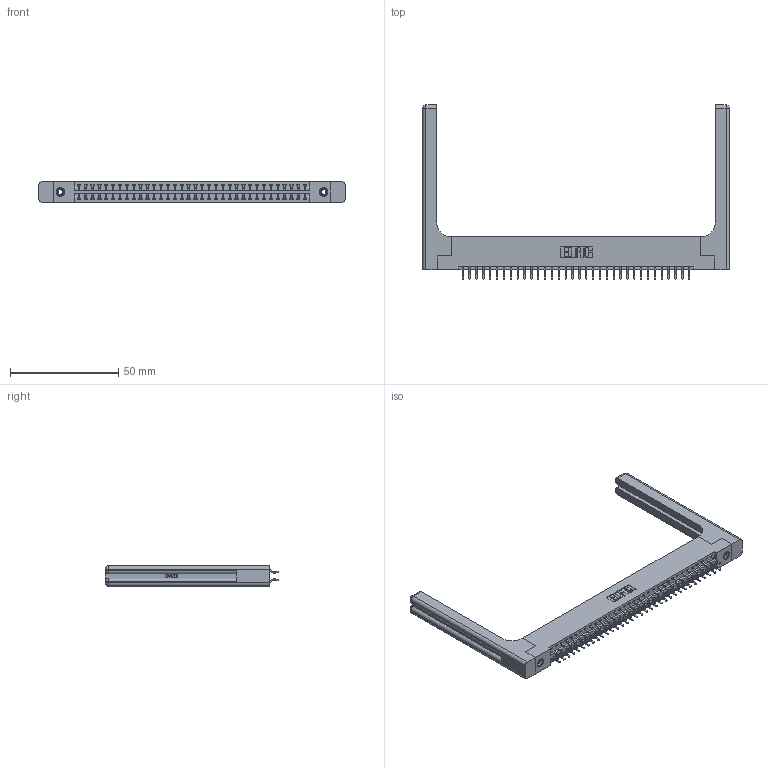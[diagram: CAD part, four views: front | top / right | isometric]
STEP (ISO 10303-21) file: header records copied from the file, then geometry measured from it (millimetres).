
FILE_DESCRIPTION (( 'STEP AP203' ), '1' );
FILE_NAME ('346-068-556-258.STEP', '2022-05-24T19:52:04', ( '' ), ( '' ), 'SwSTEP 2.0', 'SolidWorks 2020', '' );
FILE_SCHEMA (( 'CONFIG_CONTROL_DESIGN' ));
Length unit declared in the file: inch
Products named in the file (5): 346 Part_Flush Mounting Lugs - 0.156 Dia-TH; 346-068-556-258; 346-220-058_345-220-058; 345-292-001_556 Tail; 345-250-001_345-250-001-102
Assembly tree (73 placements, depth 2):
  346-068-556-258
    346 Part_Flush Mounting Lugs - 0.156 Dia-TH
    345-292-001_556 Tail  x68
    345-250-001_345-250-001-102  x2
    346-220-058_345-220-058  x2
Bounding box: 142.01 x 80.53 x 9.4 mm (x, y, z)
Volume: 21259.2 mm3; surface area: 23739.3 mm2
Topology: 73 solids, 73 shells, 4336 faces, 12795 edges, 8418 vertices
Faces by surface type: plane 2890, cylinder 1386, bspline 36, cone 12, sphere 8, torus 4
Entity records: 29084 total; most frequent: CARTESIAN_POINT 5831, ORIENTED_EDGE 4548, DIRECTION 4110, EDGE_CURVE 2274, VECTOR 1906, LINE 1906, VERTEX_POINT 1506, AXIS2_PLACEMENT_3D 1102
